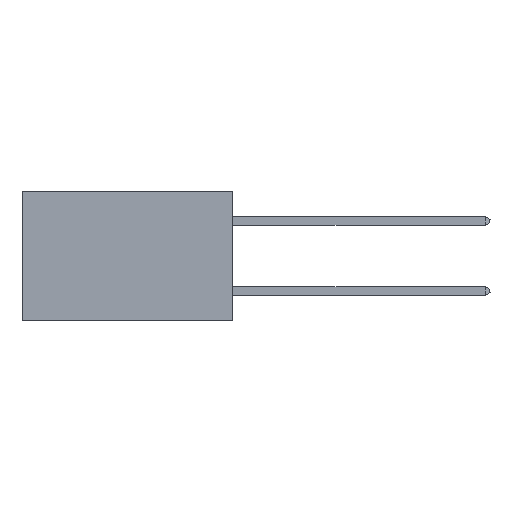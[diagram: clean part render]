
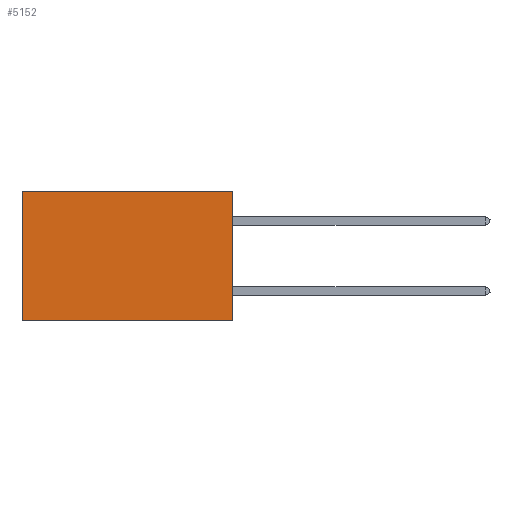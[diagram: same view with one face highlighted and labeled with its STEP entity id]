
A CAD part, left-side view. The second image highlights one B-rep face of the part: STEP entity #5152.
In plain terms, the highlighted planar face has unit normal (-1, 0, 0).
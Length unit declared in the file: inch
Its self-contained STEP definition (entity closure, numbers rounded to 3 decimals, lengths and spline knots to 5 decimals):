
#1163 = EDGE_CURVE ( 'NONE', #3632, #5969, #22692, .T. ) ;
#1987 = LINE ( 'NONE', #24981, #5875 ) ;
#2164 = CARTESIAN_POINT ( 'NONE',  ( 0.2875, 0.6, -0.37 ) ) ;
#3348 = ORIENTED_EDGE ( 'NONE', *, *, #1163, .T. ) ;
#3495 = ORIENTED_EDGE ( 'NONE', *, *, #20844, .F. ) ;
#3632 = VERTEX_POINT ( 'NONE', #7285 ) ;
#4771 = DIRECTION ( 'NONE',  ( 0., 0., -1. ) ) ;
#5152 = ADVANCED_FACE ( 'NONE', ( #8809 ), #32197, .F. ) ;
#5875 = VECTOR ( 'NONE', #4771, 39.37008 ) ;
#5969 = VERTEX_POINT ( 'NONE', #19984 ) ;
#6881 = LINE ( 'NONE', #14684, #11930 ) ;
#7285 = CARTESIAN_POINT ( 'NONE',  ( 0.2875, 0., 0. ) ) ;
#8809 = FACE_OUTER_BOUND ( 'NONE', #28758, .T. ) ;
#10574 = EDGE_CURVE ( 'NONE', #24380, #19046, #14018, .T. ) ;
#11558 = AXIS2_PLACEMENT_3D ( 'NONE', #23487, #20513, #31011 ) ;
#11930 = VECTOR ( 'NONE', #24836, 39.37008 ) ;
#14018 = LINE ( 'NONE', #19303, #16829 ) ;
#14045 = DIRECTION ( 'NONE',  ( 0., 1., 0. ) ) ;
#14684 = CARTESIAN_POINT ( 'NONE',  ( 0.2875, 0., 0. ) ) ;
#15028 = CARTESIAN_POINT ( 'NONE',  ( 0.2875, 0., -0.37 ) ) ;
#16829 = VECTOR ( 'NONE', #14045, 39.37008 ) ;
#17282 = EDGE_CURVE ( 'NONE', #5969, #19046, #1987, .T. ) ;
#19046 = VERTEX_POINT ( 'NONE', #2164 ) ;
#19303 = CARTESIAN_POINT ( 'NONE',  ( 0.2875, 0., -0.37 ) ) ;
#19984 = CARTESIAN_POINT ( 'NONE',  ( 0.2875, 0.6, 0. ) ) ;
#20513 = DIRECTION ( 'NONE',  ( 1., 0., 0. ) ) ;
#20844 = EDGE_CURVE ( 'NONE', #3632, #24380, #6881, .T. ) ;
#22692 = LINE ( 'NONE', #28689, #32085 ) ;
#23261 = DIRECTION ( 'NONE',  ( 0., 1., 0. ) ) ;
#23487 = CARTESIAN_POINT ( 'NONE',  ( 0.2875, 0., 0. ) ) ;
#23821 = ORIENTED_EDGE ( 'NONE', *, *, #10574, .F. ) ;
#24380 = VERTEX_POINT ( 'NONE', #15028 ) ;
#24836 = DIRECTION ( 'NONE',  ( 0., 0., -1. ) ) ;
#24981 = CARTESIAN_POINT ( 'NONE',  ( 0.2875, 0.6, 0. ) ) ;
#28689 = CARTESIAN_POINT ( 'NONE',  ( 0.2875, 0., 0. ) ) ;
#28758 = EDGE_LOOP ( 'NONE', ( #31770, #23821, #3495, #3348 ) ) ;
#31011 = DIRECTION ( 'NONE',  ( 0., 0., -1. ) ) ;
#31770 = ORIENTED_EDGE ( 'NONE', *, *, #17282, .T. ) ;
#32085 = VECTOR ( 'NONE', #23261, 39.37008 ) ;
#32197 = PLANE ( 'NONE',  #11558 ) ;
